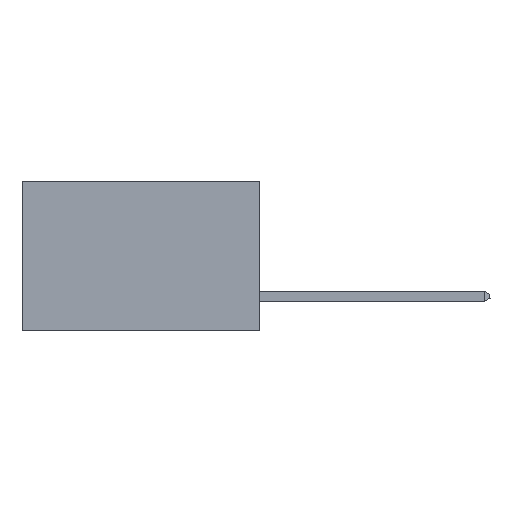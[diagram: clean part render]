
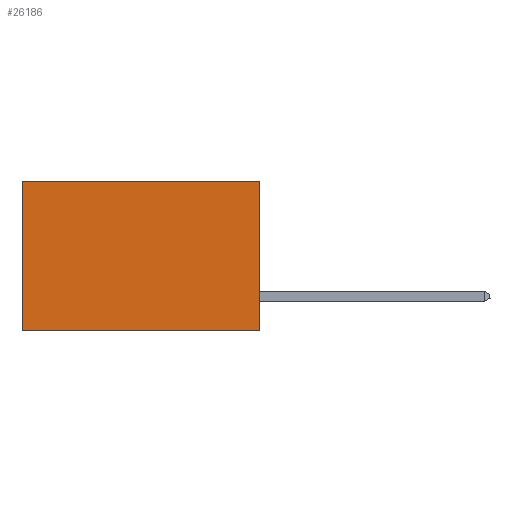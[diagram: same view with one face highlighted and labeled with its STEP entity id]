
A CAD part, left-side view. The second image highlights one B-rep face of the part: STEP entity #26186.
In plain terms, the highlighted planar face has unit normal (-1, 0, 0).
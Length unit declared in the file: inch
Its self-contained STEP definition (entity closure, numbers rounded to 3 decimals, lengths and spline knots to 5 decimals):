
#310 = ORIENTED_EDGE ( 'NONE', *, *, #21272, .F. ) ;
#1651 = CARTESIAN_POINT ( 'NONE',  ( 0.277, 0., -0.37 ) ) ;
#1689 = EDGE_CURVE ( 'NONE', #2413, #6567, #27992, .T. ) ;
#2413 = VERTEX_POINT ( 'NONE', #12600 ) ;
#5582 = VECTOR ( 'NONE', #22982, 39.37008 ) ;
#5656 = VERTEX_POINT ( 'NONE', #15974 ) ;
#6535 = VECTOR ( 'NONE', #20945, 39.37008 ) ;
#6567 = VERTEX_POINT ( 'NONE', #31906 ) ;
#6695 = PLANE ( 'NONE',  #15817 ) ;
#8425 = ORIENTED_EDGE ( 'NONE', *, *, #14201, .T. ) ;
#8704 = DIRECTION ( 'NONE',  ( 0., 0., -1. ) ) ;
#9220 = DIRECTION ( 'NONE',  ( 0., 0., -1. ) ) ;
#10559 = CARTESIAN_POINT ( 'NONE',  ( 0.277, 0., -0.37 ) ) ;
#11256 = CARTESIAN_POINT ( 'NONE',  ( 0.277, 0., 0. ) ) ;
#12039 = EDGE_CURVE ( 'NONE', #23560, #5656, #26349, .T. ) ;
#12348 = VECTOR ( 'NONE', #8704, 39.37008 ) ;
#12600 = CARTESIAN_POINT ( 'NONE',  ( 0.277, 0., 0. ) ) ;
#14201 = EDGE_CURVE ( 'NONE', #6567, #5656, #25425, .T. ) ;
#15817 = AXIS2_PLACEMENT_3D ( 'NONE', #1651, #24130, #9220 ) ;
#15974 = CARTESIAN_POINT ( 'NONE',  ( 0.277, 0.59, -0.37 ) ) ;
#18444 = CARTESIAN_POINT ( 'NONE',  ( 0.277, 0., -0.37 ) ) ;
#20502 = CARTESIAN_POINT ( 'NONE',  ( 0.277, 0.59, -0.37 ) ) ;
#20553 = EDGE_LOOP ( 'NONE', ( #8425, #22429, #310, #28673 ) ) ;
#20945 = DIRECTION ( 'NONE',  ( 0., 1., 0. ) ) ;
#21272 = EDGE_CURVE ( 'NONE', #2413, #23560, #25483, .T. ) ;
#22429 = ORIENTED_EDGE ( 'NONE', *, *, #12039, .F. ) ;
#22982 = DIRECTION ( 'NONE',  ( 0., 0., -1. ) ) ;
#23560 = VERTEX_POINT ( 'NONE', #10559 ) ;
#24130 = DIRECTION ( 'NONE',  ( 1., 0., 0. ) ) ;
#25425 = LINE ( 'NONE', #20502, #5582 ) ;
#25483 = LINE ( 'NONE', #30770, #12348 ) ;
#25627 = DIRECTION ( 'NONE',  ( 0., 1., 0. ) ) ;
#26186 = ADVANCED_FACE ( 'NONE', ( #31929 ), #6695, .F. ) ;
#26349 = LINE ( 'NONE', #18444, #6535 ) ;
#27234 = VECTOR ( 'NONE', #25627, 39.37008 ) ;
#27992 = LINE ( 'NONE', #11256, #27234 ) ;
#28673 = ORIENTED_EDGE ( 'NONE', *, *, #1689, .T. ) ;
#30770 = CARTESIAN_POINT ( 'NONE',  ( 0.277, 0., -0.37 ) ) ;
#31906 = CARTESIAN_POINT ( 'NONE',  ( 0.277, 0.59, 0. ) ) ;
#31929 = FACE_OUTER_BOUND ( 'NONE', #20553, .T. ) ;
